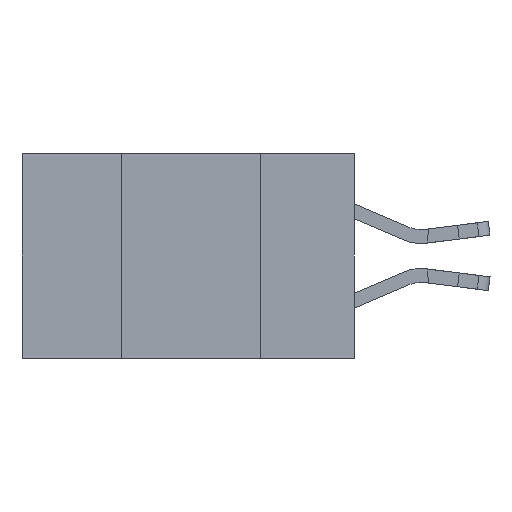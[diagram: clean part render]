
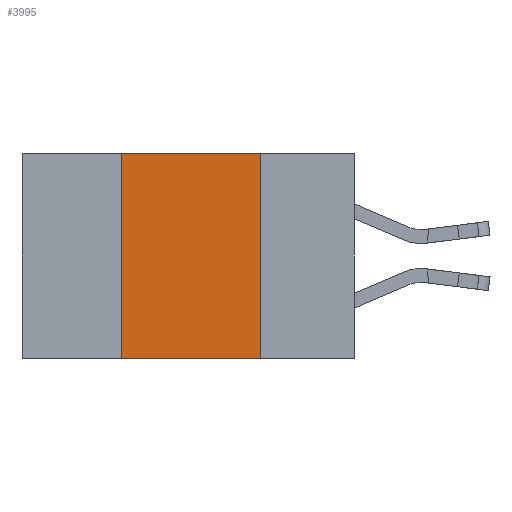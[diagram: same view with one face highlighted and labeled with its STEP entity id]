
A CAD part, left-side view. The second image highlights one B-rep face of the part: STEP entity #3995.
In plain terms, the highlighted planar face has unit normal (-1, 0, 0).
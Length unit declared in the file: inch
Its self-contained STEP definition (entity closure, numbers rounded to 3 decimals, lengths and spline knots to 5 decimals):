
#64 = ORIENTED_EDGE ( 'NONE', *, *, #16896, .F. ) ;
#744 = CARTESIAN_POINT ( 'NONE',  ( 0., 0.6, -0.37 ) ) ;
#1396 = LINE ( 'NONE', #12551, #15295 ) ;
#2398 = CARTESIAN_POINT ( 'NONE',  ( 0., 0.17, 0. ) ) ;
#3181 = VERTEX_POINT ( 'NONE', #10855 ) ;
#3336 = EDGE_CURVE ( 'NONE', #11494, #9452, #10670, .T. ) ;
#3585 = LINE ( 'NONE', #4431, #17315 ) ;
#3626 = DIRECTION ( 'NONE',  ( 0., -1., 0. ) ) ;
#3995 = ADVANCED_FACE ( 'NONE', ( #7145 ), #4432, .F. ) ;
#4232 = DIRECTION ( 'NONE',  ( 0., 0., -1. ) ) ;
#4265 = DIRECTION ( 'NONE',  ( 1., 0., 0. ) ) ;
#4354 = CARTESIAN_POINT ( 'NONE',  ( 0., 0.6, 0. ) ) ;
#4431 = CARTESIAN_POINT ( 'NONE',  ( 0., 0.42, -0.37 ) ) ;
#4432 = PLANE ( 'NONE',  #15861 ) ;
#5152 = VECTOR ( 'NONE', #3626, 39.37008 ) ;
#5895 = DIRECTION ( 'NONE',  ( 0., 0., 1. ) ) ;
#7145 = FACE_OUTER_BOUND ( 'NONE', #11244, .T. ) ;
#7912 = ORIENTED_EDGE ( 'NONE', *, *, #12666, .F. ) ;
#9229 = VERTEX_POINT ( 'NONE', #13287 ) ;
#9452 = VERTEX_POINT ( 'NONE', #2398 ) ;
#9524 = CARTESIAN_POINT ( 'NONE',  ( 0., 0.6, 0. ) ) ;
#9544 = DIRECTION ( 'NONE',  ( 0., -1., 0. ) ) ;
#10292 = ORIENTED_EDGE ( 'NONE', *, *, #3336, .F. ) ;
#10670 = LINE ( 'NONE', #9524, #11092 ) ;
#10855 = CARTESIAN_POINT ( 'NONE',  ( 0., 0.42, -0.37 ) ) ;
#11092 = VECTOR ( 'NONE', #9544, 39.37008 ) ;
#11244 = EDGE_LOOP ( 'NONE', ( #64, #10292, #7912, #14220 ) ) ;
#11494 = VERTEX_POINT ( 'NONE', #14290 ) ;
#12346 = EDGE_CURVE ( 'NONE', #3181, #9229, #12949, .T. ) ;
#12551 = CARTESIAN_POINT ( 'NONE',  ( 0., 0.17, -0.37 ) ) ;
#12666 = EDGE_CURVE ( 'NONE', #3181, #11494, #3585, .T. ) ;
#12949 = LINE ( 'NONE', #744, #5152 ) ;
#13287 = CARTESIAN_POINT ( 'NONE',  ( 0., 0.17, -0.37 ) ) ;
#14220 = ORIENTED_EDGE ( 'NONE', *, *, #12346, .T. ) ;
#14290 = CARTESIAN_POINT ( 'NONE',  ( 0., 0.42, 0. ) ) ;
#15248 = DIRECTION ( 'NONE',  ( 0., 0., -1. ) ) ;
#15295 = VECTOR ( 'NONE', #15248, 39.37008 ) ;
#15861 = AXIS2_PLACEMENT_3D ( 'NONE', #4354, #4265, #4232 ) ;
#16896 = EDGE_CURVE ( 'NONE', #9452, #9229, #1396, .T. ) ;
#17315 = VECTOR ( 'NONE', #5895, 39.37008 ) ;
